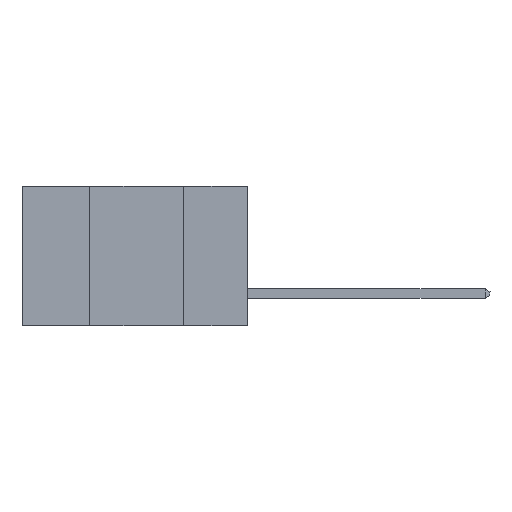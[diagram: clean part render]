
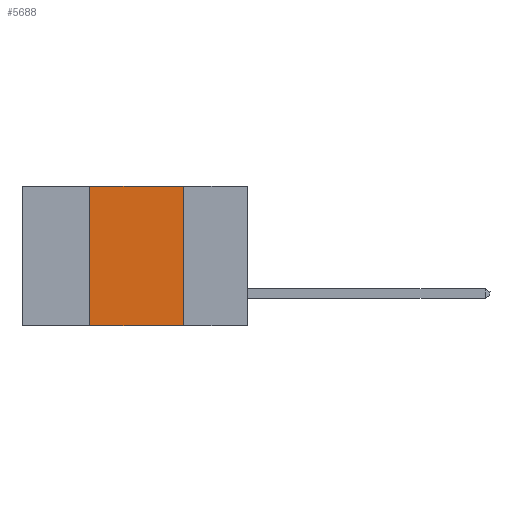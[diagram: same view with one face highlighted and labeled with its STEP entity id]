
A CAD part, left-side view. The second image highlights one B-rep face of the part: STEP entity #5688.
In plain terms, the highlighted planar face has unit normal (-1, 0, 0).
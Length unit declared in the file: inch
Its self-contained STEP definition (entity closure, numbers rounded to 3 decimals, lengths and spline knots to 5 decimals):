
#210 = DIRECTION ( 'NONE',  ( 0., -1., 0. ) ) ;
#336 = VECTOR ( 'NONE', #9016, 39.37008 ) ;
#536 = ORIENTED_EDGE ( 'NONE', *, *, #3717, .F. ) ;
#1347 = VERTEX_POINT ( 'NONE', #1751 ) ;
#1370 = LINE ( 'NONE', #3098, #4767 ) ;
#1376 = VERTEX_POINT ( 'NONE', #5974 ) ;
#1666 = ORIENTED_EDGE ( 'NONE', *, *, #10256, .F. ) ;
#1751 = CARTESIAN_POINT ( 'NONE',  ( 0., 0.42, 0. ) ) ;
#2217 = EDGE_LOOP ( 'NONE', ( #536, #1666, #6822, #3560 ) ) ;
#2483 = CARTESIAN_POINT ( 'NONE',  ( 0., 0.17, 0. ) ) ;
#2551 = LINE ( 'NONE', #7885, #8077 ) ;
#3098 = CARTESIAN_POINT ( 'NONE',  ( 0., 0.42, -0.37 ) ) ;
#3335 = VERTEX_POINT ( 'NONE', #10323 ) ;
#3560 = ORIENTED_EDGE ( 'NONE', *, *, #9114, .T. ) ;
#3717 = EDGE_CURVE ( 'NONE', #4239, #1376, #2551, .T. ) ;
#4005 = FACE_OUTER_BOUND ( 'NONE', #2217, .T. ) ;
#4176 = DIRECTION ( 'NONE',  ( 1., 0., 0. ) ) ;
#4239 = VERTEX_POINT ( 'NONE', #2483 ) ;
#4767 = VECTOR ( 'NONE', #6536, 39.37008 ) ;
#4776 = VECTOR ( 'NONE', #210, 39.37008 ) ;
#5202 = DIRECTION ( 'NONE',  ( 0., 0., -1. ) ) ;
#5347 = LINE ( 'NONE', #7918, #4776 ) ;
#5688 = ADVANCED_FACE ( 'NONE', ( #4005 ), #10052, .F. ) ;
#5974 = CARTESIAN_POINT ( 'NONE',  ( 0., 0.17, -0.37 ) ) ;
#6536 = DIRECTION ( 'NONE',  ( 0., 0., 1. ) ) ;
#6580 = DIRECTION ( 'NONE',  ( 0., 0., -1. ) ) ;
#6822 = ORIENTED_EDGE ( 'NONE', *, *, #8896, .F. ) ;
#7885 = CARTESIAN_POINT ( 'NONE',  ( 0., 0.17, -0.37 ) ) ;
#7918 = CARTESIAN_POINT ( 'NONE',  ( 0., 0.6, -0.37 ) ) ;
#8064 = CARTESIAN_POINT ( 'NONE',  ( 0., 0.6, 0. ) ) ;
#8077 = VECTOR ( 'NONE', #5202, 39.37008 ) ;
#8429 = CARTESIAN_POINT ( 'NONE',  ( 0., 0.6, 0. ) ) ;
#8644 = AXIS2_PLACEMENT_3D ( 'NONE', #8429, #4176, #6580 ) ;
#8896 = EDGE_CURVE ( 'NONE', #3335, #1347, #1370, .T. ) ;
#9016 = DIRECTION ( 'NONE',  ( 0., -1., 0. ) ) ;
#9114 = EDGE_CURVE ( 'NONE', #3335, #1376, #5347, .T. ) ;
#9854 = LINE ( 'NONE', #8064, #336 ) ;
#10052 = PLANE ( 'NONE',  #8644 ) ;
#10256 = EDGE_CURVE ( 'NONE', #1347, #4239, #9854, .T. ) ;
#10323 = CARTESIAN_POINT ( 'NONE',  ( 0., 0.42, -0.37 ) ) ;
